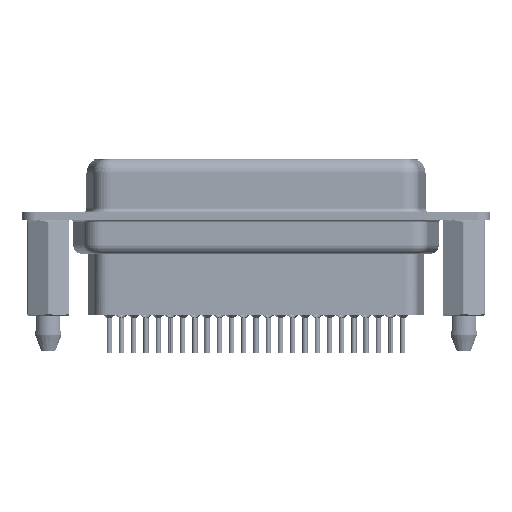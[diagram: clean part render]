
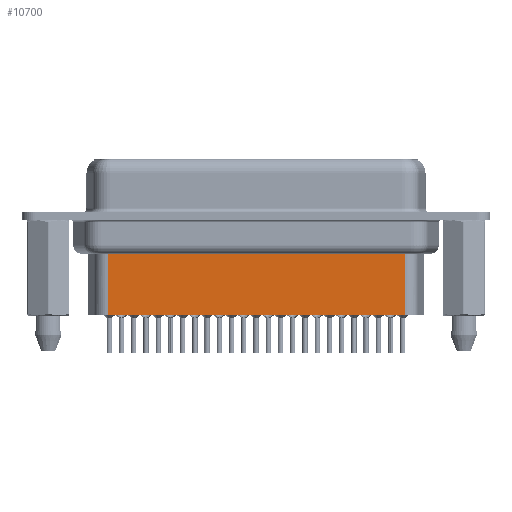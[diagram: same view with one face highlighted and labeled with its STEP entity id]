
A CAD part, front view. The second image highlights one B-rep face of the part: STEP entity #10700.
In plain terms, the highlighted planar face has unit normal (0, -1, 0).
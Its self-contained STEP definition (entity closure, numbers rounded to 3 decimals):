
#455 = EDGE_CURVE ( 'NONE', #9682, #7872, #30676, .T. ) ;
#846 = LINE ( 'NONE', #5174, #9161 ) ;
#1260 = DIRECTION ( 'NONE',  ( 1., 0., 0. ) ) ;
#2734 = EDGE_CURVE ( 'NONE', #9682, #4526, #846, .T. ) ;
#3924 = CARTESIAN_POINT ( 'NONE',  ( 6.459, -3.5, -4.097 ) ) ;
#4526 = VERTEX_POINT ( 'NONE', #13283 ) ;
#5166 = CARTESIAN_POINT ( 'NONE',  ( 6.706, -3.5, -3.1 ) ) ;
#5174 = CARTESIAN_POINT ( 'NONE',  ( 40.344, -3.5, -3.1 ) ) ;
#5898 = PLANE ( 'NONE',  #14250 ) ;
#6786 = ORIENTED_EDGE ( 'NONE', *, *, #2734, .F. ) ;
#7872 = VERTEX_POINT ( 'NONE', #16612 ) ;
#8190 = LINE ( 'NONE', #5166, #22418 ) ;
#8957 = VERTEX_POINT ( 'NONE', #9587 ) ;
#9161 = VECTOR ( 'NONE', #15069, 1000. ) ;
#9587 = CARTESIAN_POINT ( 'NONE',  ( 6.706, -3.5, -11.15 ) ) ;
#9682 = VERTEX_POINT ( 'NONE', #17497 ) ;
#10700 = ADVANCED_FACE ( 'NONE', ( #27821 ), #5898, .T. ) ;
#12415 = CARTESIAN_POINT ( 'NONE',  ( 6.706, -3.5, -11.15 ) ) ;
#12455 = VECTOR ( 'NONE', #21196, 1000. ) ;
#13283 = CARTESIAN_POINT ( 'NONE',  ( 40.344, -3.5, -11.15 ) ) ;
#14250 = AXIS2_PLACEMENT_3D ( 'NONE', #27972, #30716, #1260 ) ;
#15069 = DIRECTION ( 'NONE',  ( 0., 0., -1. ) ) ;
#16612 = CARTESIAN_POINT ( 'NONE',  ( 6.706, -3.5, -4.097 ) ) ;
#17497 = CARTESIAN_POINT ( 'NONE',  ( 40.344, -3.5, -4.097 ) ) ;
#20060 = LINE ( 'NONE', #12415, #29523 ) ;
#21196 = DIRECTION ( 'NONE',  ( -1., 0., 0. ) ) ;
#21399 = ORIENTED_EDGE ( 'NONE', *, *, #28091, .T. ) ;
#21752 = ORIENTED_EDGE ( 'NONE', *, *, #26306, .F. ) ;
#22418 = VECTOR ( 'NONE', #22728, 1000. ) ;
#22728 = DIRECTION ( 'NONE',  ( 0., 0., -1. ) ) ;
#25176 = DIRECTION ( 'NONE',  ( -1., 0., 0. ) ) ;
#26031 = EDGE_LOOP ( 'NONE', ( #6786, #27344, #21399, #21752 ) ) ;
#26306 = EDGE_CURVE ( 'NONE', #4526, #8957, #20060, .T. ) ;
#27344 = ORIENTED_EDGE ( 'NONE', *, *, #455, .T. ) ;
#27821 = FACE_OUTER_BOUND ( 'NONE', #26031, .T. ) ;
#27972 = CARTESIAN_POINT ( 'NONE',  ( 6.706, -3.5, -3.1 ) ) ;
#28091 = EDGE_CURVE ( 'NONE', #7872, #8957, #8190, .T. ) ;
#29523 = VECTOR ( 'NONE', #25176, 1000. ) ;
#30676 = LINE ( 'NONE', #3924, #12455 ) ;
#30716 = DIRECTION ( 'NONE',  ( 0., -1., 0. ) ) ;
